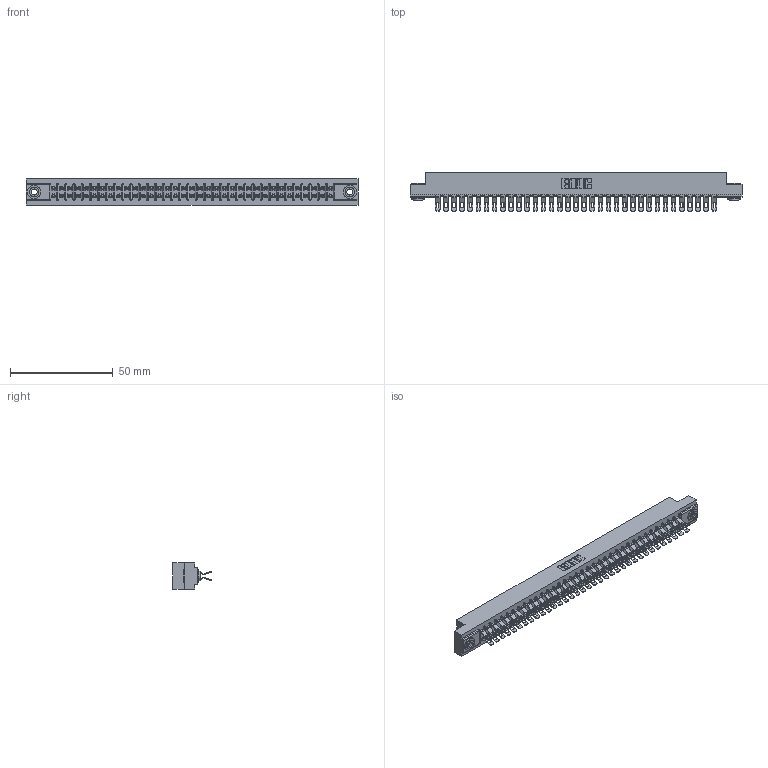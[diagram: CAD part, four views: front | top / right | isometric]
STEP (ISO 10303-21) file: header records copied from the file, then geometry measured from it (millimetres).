
FILE_DESCRIPTION (( 'STEP AP203' ), '1' );
FILE_NAME ('307-070-455-203.STEP', '2020-10-01T00:25:51', ( '' ), ( '' ), 'SwSTEP 2.0', 'SolidWorks 2020', '' );
FILE_SCHEMA (( 'CONFIG_CONTROL_DESIGN' ));
Length unit declared in the file: inch
Products named in the file (4): 345-250-002_345-250-002-102; 307-290-001_555; 307 Part_.156 Dia Mounting Holes; 307-070-455-203
Assembly tree (73 placements, depth 2):
  307-070-455-203
    307 Part_.156 Dia Mounting Holes
    307-290-001_555  x70
    345-250-002_345-250-002-102  x2
Bounding box: 161.7 x 18.75 x 12.7 mm (x, y, z)
Volume: 17354.8 mm3; surface area: 22501.3 mm2
Topology: 73 solids, 73 shells, 4476 faces, 13105 edges, 8542 vertices
Faces by surface type: plane 2474, cylinder 1922, sphere 72, cone 8
Entity records: 33590 total; most frequent: CARTESIAN_POINT 5484, ORIENTED_EDGE 5428, DIRECTION 5396, EDGE_CURVE 2714, VECTOR 2060, LINE 2060, VERTEX_POINT 1756, AXIS2_PLACEMENT_3D 1668
